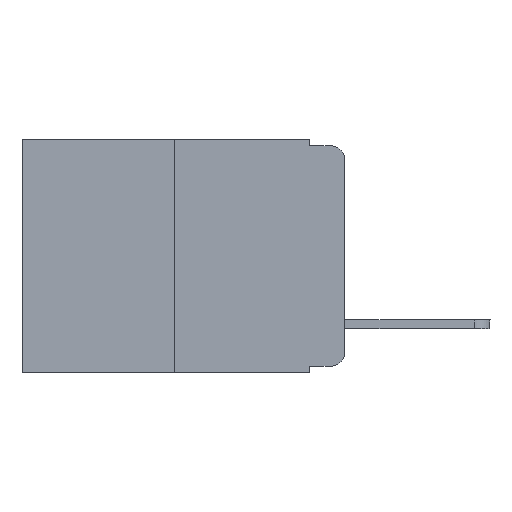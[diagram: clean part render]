
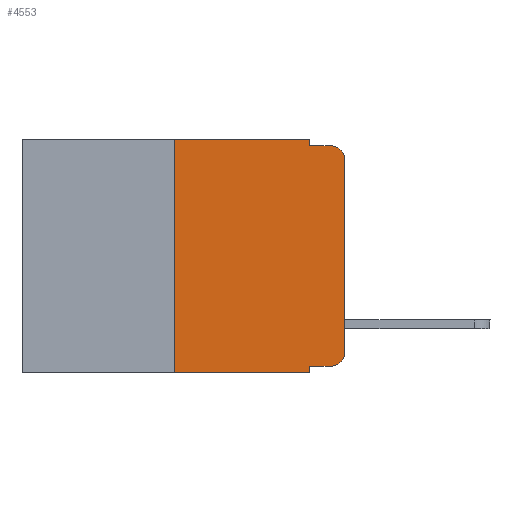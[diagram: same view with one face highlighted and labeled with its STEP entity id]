
A CAD part, left-side view. The second image highlights one B-rep face of the part: STEP entity #4553.
In plain terms, the highlighted planar face has unit normal (-1, 0, 0).
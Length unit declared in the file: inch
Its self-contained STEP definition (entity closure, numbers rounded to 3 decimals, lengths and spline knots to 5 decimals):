
#206 = CIRCLE ( 'NONE', #14379, 0.02 ) ;
#216 = CARTESIAN_POINT ( 'NONE',  ( 0., 0.051, -0.01 ) ) ;
#782 = VECTOR ( 'NONE', #22590, 39.37008 ) ;
#962 = VERTEX_POINT ( 'NONE', #5704 ) ;
#1018 = VERTEX_POINT ( 'NONE', #6118 ) ;
#1299 = EDGE_CURVE ( 'NONE', #962, #16743, #19327, .T. ) ;
#1759 = LINE ( 'NONE', #23044, #10472 ) ;
#1838 = VECTOR ( 'NONE', #3211, 39.37008 ) ;
#2371 = EDGE_CURVE ( 'NONE', #1018, #8261, #206, .T. ) ;
#2454 = VECTOR ( 'NONE', #12346, 39.37008 ) ;
#2507 = CARTESIAN_POINT ( 'NONE',  ( 0., 0.02, -0.03 ) ) ;
#2545 = DIRECTION ( 'NONE',  ( -1., 0., 0. ) ) ;
#2974 = ORIENTED_EDGE ( 'NONE', *, *, #6464, .F. ) ;
#2997 = LINE ( 'NONE', #216, #2454 ) ;
#3032 = ORIENTED_EDGE ( 'NONE', *, *, #4228, .F. ) ;
#3211 = DIRECTION ( 'NONE',  ( 0., 0., 1. ) ) ;
#3280 = DIRECTION ( 'NONE',  ( 0., 0., -1. ) ) ;
#3305 = DIRECTION ( 'NONE',  ( 0., 0., 1. ) ) ;
#4228 = EDGE_CURVE ( 'NONE', #23131, #8261, #2997, .T. ) ;
#4304 = DIRECTION ( 'NONE',  ( 0., 0., -1. ) ) ;
#4553 = ADVANCED_FACE ( 'NONE', ( #7764 ), #19324, .F. ) ;
#4720 = ORIENTED_EDGE ( 'NONE', *, *, #11914, .T. ) ;
#4960 = VECTOR ( 'NONE', #3305, 39.37008 ) ;
#5327 = DIRECTION ( 'NONE',  ( 0., 0., -1. ) ) ;
#5704 = CARTESIAN_POINT ( 'NONE',  ( 0., 0.02, -0.333 ) ) ;
#6118 = CARTESIAN_POINT ( 'NONE',  ( 0., 0., -0.03 ) ) ;
#6155 = VERTEX_POINT ( 'NONE', #17396 ) ;
#6224 = DIRECTION ( 'NONE',  ( 0., 0., -1. ) ) ;
#6464 = EDGE_CURVE ( 'NONE', #16891, #23131, #1759, .T. ) ;
#6525 = VECTOR ( 'NONE', #7092, 39.37008 ) ;
#6671 = LINE ( 'NONE', #16264, #4960 ) ;
#6695 = CARTESIAN_POINT ( 'NONE',  ( 0., 0., 0. ) ) ;
#6796 = ORIENTED_EDGE ( 'NONE', *, *, #7959, .F. ) ;
#6911 = CARTESIAN_POINT ( 'NONE',  ( 0., 0.473, 0. ) ) ;
#7092 = DIRECTION ( 'NONE',  ( 0., -1., 0. ) ) ;
#7169 = ORIENTED_EDGE ( 'NONE', *, *, #20084, .F. ) ;
#7335 = LINE ( 'NONE', #12410, #6525 ) ;
#7689 = VECTOR ( 'NONE', #10011, 39.37008 ) ;
#7756 = VECTOR ( 'NONE', #5327, 39.37008 ) ;
#7764 = FACE_OUTER_BOUND ( 'NONE', #14084, .T. ) ;
#7959 = EDGE_CURVE ( 'NONE', #12865, #16891, #7335, .T. ) ;
#8261 = VERTEX_POINT ( 'NONE', #23161 ) ;
#8911 = DIRECTION ( 'NONE',  ( 1., 0., 0. ) ) ;
#8958 = CARTESIAN_POINT ( 'NONE',  ( 0., 0.25, -0.343 ) ) ;
#8992 = AXIS2_PLACEMENT_3D ( 'NONE', #11977, #2545, #6224 ) ;
#9943 = ORIENTED_EDGE ( 'NONE', *, *, #22067, .T. ) ;
#10011 = DIRECTION ( 'NONE',  ( 0., -1., 0. ) ) ;
#10472 = VECTOR ( 'NONE', #16735, 39.37008 ) ;
#10682 = CARTESIAN_POINT ( 'NONE',  ( 0., 0.25, 0. ) ) ;
#11442 = LINE ( 'NONE', #18973, #782 ) ;
#11485 = AXIS2_PLACEMENT_3D ( 'NONE', #6911, #8911, #3280 ) ;
#11914 = EDGE_CURVE ( 'NONE', #13167, #962, #11442, .T. ) ;
#11977 = CARTESIAN_POINT ( 'NONE',  ( 0., 0.02, -0.313 ) ) ;
#12245 = LINE ( 'NONE', #6695, #1838 ) ;
#12346 = DIRECTION ( 'NONE',  ( 0., -1., 0. ) ) ;
#12410 = CARTESIAN_POINT ( 'NONE',  ( 0., 0.473, 0. ) ) ;
#12498 = LINE ( 'NONE', #14143, #7756 ) ;
#12865 = VERTEX_POINT ( 'NONE', #10682 ) ;
#13167 = VERTEX_POINT ( 'NONE', #17216 ) ;
#13562 = CARTESIAN_POINT ( 'NONE',  ( 0., 0.473, -0.343 ) ) ;
#14045 = ORIENTED_EDGE ( 'NONE', *, *, #19882, .T. ) ;
#14084 = EDGE_LOOP ( 'NONE', ( #14045, #14127, #3032, #2974, #6796, #22219, #9943, #7169, #4720, #16662 ) ) ;
#14090 = LINE ( 'NONE', #13562, #7689 ) ;
#14127 = ORIENTED_EDGE ( 'NONE', *, *, #2371, .T. ) ;
#14143 = CARTESIAN_POINT ( 'NONE',  ( 0., 0.051, 0. ) ) ;
#14379 = AXIS2_PLACEMENT_3D ( 'NONE', #2507, #14983, #4304 ) ;
#14983 = DIRECTION ( 'NONE',  ( -1., 0., 0. ) ) ;
#16264 = CARTESIAN_POINT ( 'NONE',  ( 0., 0.25, 0. ) ) ;
#16662 = ORIENTED_EDGE ( 'NONE', *, *, #1299, .T. ) ;
#16735 = DIRECTION ( 'NONE',  ( 0., 0., -1. ) ) ;
#16743 = VERTEX_POINT ( 'NONE', #19758 ) ;
#16804 = CARTESIAN_POINT ( 'NONE',  ( 0., 0.051, -0.01 ) ) ;
#16891 = VERTEX_POINT ( 'NONE', #22098 ) ;
#17216 = CARTESIAN_POINT ( 'NONE',  ( 0., 0.051, -0.333 ) ) ;
#17396 = CARTESIAN_POINT ( 'NONE',  ( 0., 0.051, -0.343 ) ) ;
#18973 = CARTESIAN_POINT ( 'NONE',  ( 0., 0.051, -0.333 ) ) ;
#19324 = PLANE ( 'NONE',  #11485 ) ;
#19327 = CIRCLE ( 'NONE', #8992, 0.02 ) ;
#19527 = EDGE_CURVE ( 'NONE', #20751, #12865, #6671, .T. ) ;
#19758 = CARTESIAN_POINT ( 'NONE',  ( 0., 0., -0.313 ) ) ;
#19882 = EDGE_CURVE ( 'NONE', #16743, #1018, #12245, .T. ) ;
#20084 = EDGE_CURVE ( 'NONE', #13167, #6155, #12498, .T. ) ;
#20751 = VERTEX_POINT ( 'NONE', #8958 ) ;
#22067 = EDGE_CURVE ( 'NONE', #20751, #6155, #14090, .T. ) ;
#22098 = CARTESIAN_POINT ( 'NONE',  ( 0., 0.051, 0. ) ) ;
#22219 = ORIENTED_EDGE ( 'NONE', *, *, #19527, .F. ) ;
#22590 = DIRECTION ( 'NONE',  ( 0., -1., 0. ) ) ;
#23044 = CARTESIAN_POINT ( 'NONE',  ( 0., 0.051, 0. ) ) ;
#23131 = VERTEX_POINT ( 'NONE', #16804 ) ;
#23161 = CARTESIAN_POINT ( 'NONE',  ( 0., 0.02, -0.01 ) ) ;
